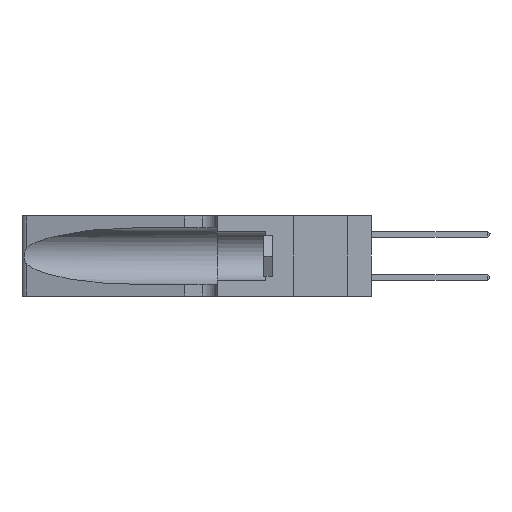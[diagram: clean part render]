
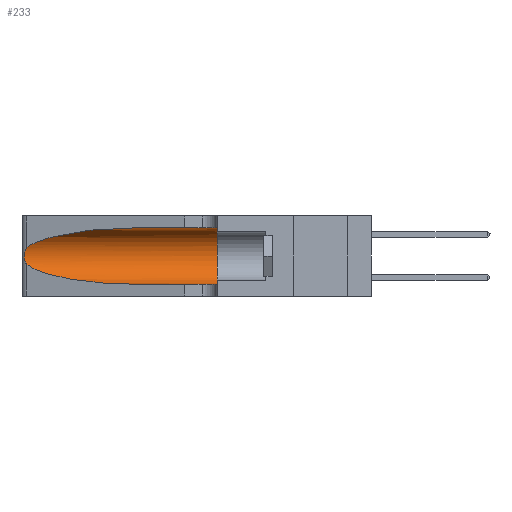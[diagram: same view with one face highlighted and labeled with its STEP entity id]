
A CAD part, left-side view. The second image highlights one B-rep face of the part: STEP entity #233.
In plain terms, the highlighted cylindrical face has radius 3.308 mm (diameter 6.617 mm), a partial arc.
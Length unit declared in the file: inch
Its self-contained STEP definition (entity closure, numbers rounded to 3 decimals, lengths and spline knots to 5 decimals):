
#182 = DIRECTION ( 'NONE',  ( 0., -1., 0. ) ) ;
#233 = ADVANCED_FACE ( 'NONE', ( #18814 ), #9990, .F. ) ;
#250 = LINE ( 'NONE', #18120, #8664 ) ;
#452 = CIRCLE ( 'NONE', #2877, 0.13025 ) ;
#501 = ORIENTED_EDGE ( 'NONE', *, *, #2815, .T. ) ;
#1161 = EDGE_LOOP ( 'NONE', ( #21526, #501, #7208, #19504, #12303, #19451 ) ) ;
#1278 = CARTESIAN_POINT ( 'NONE',  ( 0.1305, 0.72297, 0.05475 ) ) ;
#1687 = CARTESIAN_POINT ( 'NONE',  ( 0.1305, 0.72297, 0.31525 ) ) ;
#2710 = EDGE_CURVE ( 'NONE', #10894, #15513, #452, .T. ) ;
#2792 = CARTESIAN_POINT ( 'NONE',  ( 0.25639, 1.23186, 0.15144 ) ) ;
#2815 = EDGE_CURVE ( 'NONE', #13958, #10871, #19938, .T. ) ;
#2877 = AXIS2_PLACEMENT_3D ( 'NONE', #20613, #19562, #8684 ) ;
#3055 = CARTESIAN_POINT ( 'NONE',  ( 0.25487, 1.22718, 0.14631 ) ) ;
#4160 = VERTEX_POINT ( 'NONE', #1687 ) ;
#4217 = AXIS2_PLACEMENT_3D ( 'NONE', #10248, #13832, #20535 ) ;
#4366 = CARTESIAN_POINT ( 'NONE',  ( 0.25487, 1.22718, 0.14631 ) ) ;
#5089 =( BOUNDED_CURVE ( )  B_SPLINE_CURVE ( 3, ( #20079, #20229, #11888, #8489 ),
 .UNSPECIFIED., .F., .F. ) 
 B_SPLINE_CURVE_WITH_KNOTS ( ( 4, 4 ),
 ( 1.5708, 2.84003 ),
 .UNSPECIFIED. ) 
 CURVE ( )  GEOMETRIC_REPRESENTATION_ITEM ( )  RATIONAL_B_SPLINE_CURVE ( ( 1., 0.87, 0.87, 1. ) ) 
 REPRESENTATION_ITEM ( '' )  );
#5513 = VECTOR ( 'NONE', #17358, 39.37008 ) ;
#6208 = VERTEX_POINT ( 'NONE', #18022 ) ;
#6364 = CARTESIAN_POINT ( 'NONE',  ( 0.26075, 1.23896, 0.19203 ) ) ;
#7208 = ORIENTED_EDGE ( 'NONE', *, *, #13633, .T. ) ;
#7624 = CARTESIAN_POINT ( 'NONE',  ( 0.1305, 1.61858, 0.31525 ) ) ;
#7898 = CARTESIAN_POINT ( 'NONE',  ( 0.26017, 1.23833, 0.17102 ) ) ;
#7925 = CARTESIAN_POINT ( 'NONE',  ( 0.2373, 1.15595, 0.08982 ) ) ;
#8489 = CARTESIAN_POINT ( 'NONE',  ( 0.25487, 1.22718, 0.22369 ) ) ;
#8664 = VECTOR ( 'NONE', #182, 39.37008 ) ;
#8684 = DIRECTION ( 'NONE',  ( 0., 0., 1. ) ) ;
#9278 = CARTESIAN_POINT ( 'NONE',  ( 0.25854, 1.2359, 0.20912 ) ) ;
#9626 = CARTESIAN_POINT ( 'NONE',  ( 0.25555, 1.22993, 0.14849 ) ) ;
#9926 = EDGE_CURVE ( 'NONE', #4160, #10894, #17706, .T. ) ;
#9990 = CYLINDRICAL_SURFACE ( 'NONE', #4217, 0.13025 ) ;
#10248 = CARTESIAN_POINT ( 'NONE',  ( 0.1305, 1.61858, 0.185 ) ) ;
#10871 = VERTEX_POINT ( 'NONE', #3055 ) ;
#10894 = VERTEX_POINT ( 'NONE', #19886 ) ;
#11234 = CARTESIAN_POINT ( 'NONE',  ( 0.25856, 1.23593, 0.16098 ) ) ;
#11888 = CARTESIAN_POINT ( 'NONE',  ( 0.2373, 1.15595, 0.28018 ) ) ;
#12303 = ORIENTED_EDGE ( 'NONE', *, *, #2710, .F. ) ;
#12380 = CARTESIAN_POINT ( 'NONE',  ( 0.26018, 1.23835, 0.19895 ) ) ;
#13633 = EDGE_CURVE ( 'NONE', #10871, #6208, #16688, .T. ) ;
#13832 = DIRECTION ( 'NONE',  ( 0., -1., 0. ) ) ;
#13958 = VERTEX_POINT ( 'NONE', #20376 ) ;
#14312 = CARTESIAN_POINT ( 'NONE',  ( 0.26075, 1.23896, 0.178 ) ) ;
#15067 = CARTESIAN_POINT ( 'NONE',  ( 0.25487, 1.22718, 0.22369 ) ) ;
#15134 = CARTESIAN_POINT ( 'NONE',  ( 0.1305, 0.35, 0.05475 ) ) ;
#15141 = CARTESIAN_POINT ( 'NONE',  ( 0.25555, 1.22994, 0.2215 ) ) ;
#15513 = VERTEX_POINT ( 'NONE', #15134 ) ;
#15698 = EDGE_CURVE ( 'NONE', #6208, #15513, #250, .T. ) ;
#16688 =( BOUNDED_CURVE ( )  B_SPLINE_CURVE ( 3, ( #17848, #7925, #17696, #1278 ),
 .UNSPECIFIED., .F., .F. ) 
 B_SPLINE_CURVE_WITH_KNOTS ( ( 4, 4 ),
 ( 3.44316, 4.71239 ),
 .UNSPECIFIED. ) 
 CURVE ( )  GEOMETRIC_REPRESENTATION_ITEM ( )  RATIONAL_B_SPLINE_CURVE ( ( 1., 0.87, 0.87, 1. ) ) 
 REPRESENTATION_ITEM ( '' )  );
#17358 = DIRECTION ( 'NONE',  ( 0., -1., 0. ) ) ;
#17696 = CARTESIAN_POINT ( 'NONE',  ( 0.18966, 0.96281, 0.05475 ) ) ;
#17706 = LINE ( 'NONE', #7624, #5513 ) ;
#17849 = EDGE_CURVE ( 'NONE', #4160, #13958, #5089, .T. ) ;
#17848 = CARTESIAN_POINT ( 'NONE',  ( 0.25487, 1.22718, 0.14631 ) ) ;
#18022 = CARTESIAN_POINT ( 'NONE',  ( 0.1305, 0.72297, 0.05475 ) ) ;
#18120 = CARTESIAN_POINT ( 'NONE',  ( 0.1305, 1.61858, 0.05475 ) ) ;
#18814 = FACE_OUTER_BOUND ( 'NONE', #1161, .T. ) ;
#19451 = ORIENTED_EDGE ( 'NONE', *, *, #9926, .F. ) ;
#19504 = ORIENTED_EDGE ( 'NONE', *, *, #15698, .T. ) ;
#19562 = DIRECTION ( 'NONE',  ( 0., 1., 0. ) ) ;
#19886 = CARTESIAN_POINT ( 'NONE',  ( 0.1305, 0.35, 0.31525 ) ) ;
#19938 = B_SPLINE_CURVE_WITH_KNOTS ( 'NONE', 3,
 ( #15067, #15141, #20240, #20746, #9278, #12380, #6364, #14312, #7898, #11234, #21093, #2792, #9626, #4366 ),
 .UNSPECIFIED., .F., .F.,
 ( 4, 2, 2, 2, 2, 2, 4 ),
 ( 0., 0.00027, 0.00053, 0.00107, 0.0016, 0.00187, 0.00214 ),
 .UNSPECIFIED. ) ;
#20079 = CARTESIAN_POINT ( 'NONE',  ( 0.1305, 0.72297, 0.31525 ) ) ;
#20229 = CARTESIAN_POINT ( 'NONE',  ( 0.18966, 0.96281, 0.31525 ) ) ;
#20240 = CARTESIAN_POINT ( 'NONE',  ( 0.25639, 1.23184, 0.21858 ) ) ;
#20376 = CARTESIAN_POINT ( 'NONE',  ( 0.25487, 1.22718, 0.22369 ) ) ;
#20535 = DIRECTION ( 'NONE',  ( 0., 0., -1. ) ) ;
#20613 = CARTESIAN_POINT ( 'NONE',  ( 0.1305, 0.35, 0.185 ) ) ;
#20746 = CARTESIAN_POINT ( 'NONE',  ( 0.25787, 1.23484, 0.2124 ) ) ;
#21093 = CARTESIAN_POINT ( 'NONE',  ( 0.25789, 1.23486, 0.15765 ) ) ;
#21526 = ORIENTED_EDGE ( 'NONE', *, *, #17849, .T. ) ;
